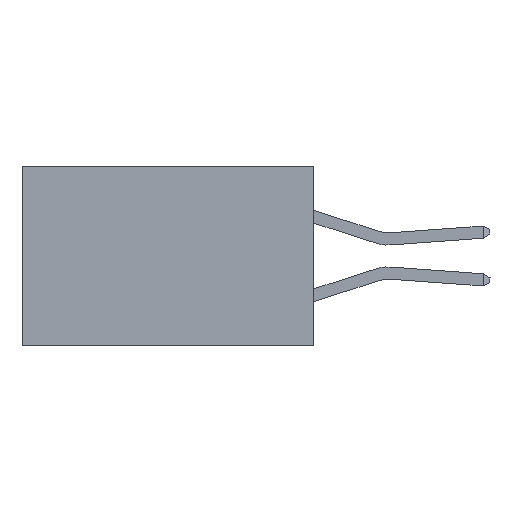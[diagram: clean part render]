
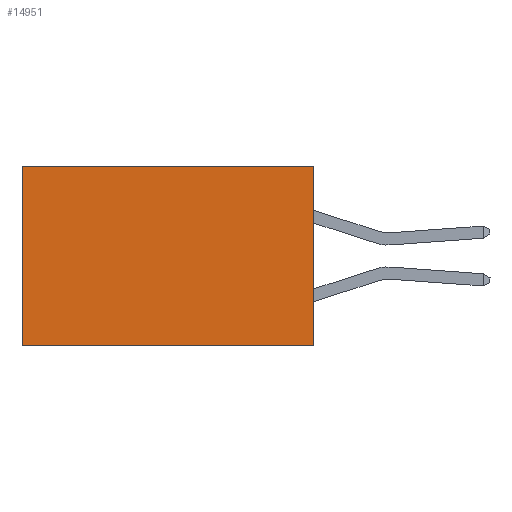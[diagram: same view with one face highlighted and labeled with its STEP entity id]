
A CAD part, left-side view. The second image highlights one B-rep face of the part: STEP entity #14951.
In plain terms, the highlighted planar face has unit normal (-1, 0, 0).
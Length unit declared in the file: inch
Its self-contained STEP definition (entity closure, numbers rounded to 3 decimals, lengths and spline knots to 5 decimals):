
#868 = FACE_OUTER_BOUND ( 'NONE', #6961, .T. ) ;
#1826 = PLANE ( 'NONE',  #11063 ) ;
#2265 = LINE ( 'NONE', #15560, #13310 ) ;
#2710 = ORIENTED_EDGE ( 'NONE', *, *, #5922, .T. ) ;
#3323 = VECTOR ( 'NONE', #17040, 39.37008 ) ;
#3349 = CARTESIAN_POINT ( 'NONE',  ( 0.2875, 0., 0. ) ) ;
#3392 = VERTEX_POINT ( 'NONE', #16728 ) ;
#4278 = VERTEX_POINT ( 'NONE', #12067 ) ;
#4485 = CARTESIAN_POINT ( 'NONE',  ( 0.2875, 0.6, 0. ) ) ;
#5289 = VECTOR ( 'NONE', #5847, 39.37008 ) ;
#5847 = DIRECTION ( 'NONE',  ( 0., 0., -1. ) ) ;
#5922 = EDGE_CURVE ( 'NONE', #6844, #16565, #13421, .T. ) ;
#6163 = DIRECTION ( 'NONE',  ( 1., 0., 0. ) ) ;
#6703 = VECTOR ( 'NONE', #11893, 39.37008 ) ;
#6844 = VERTEX_POINT ( 'NONE', #12405 ) ;
#6961 = EDGE_LOOP ( 'NONE', ( #2710, #13557, #9890, #16768 ) ) ;
#9796 = EDGE_CURVE ( 'NONE', #4278, #3392, #2265, .T. ) ;
#9890 = ORIENTED_EDGE ( 'NONE', *, *, #9796, .F. ) ;
#11063 = AXIS2_PLACEMENT_3D ( 'NONE', #3349, #6163, #16149 ) ;
#11360 = EDGE_CURVE ( 'NONE', #4278, #6844, #17961, .T. ) ;
#11893 = DIRECTION ( 'NONE',  ( 0., 1., 0. ) ) ;
#12067 = CARTESIAN_POINT ( 'NONE',  ( 0.2875, 0., 0. ) ) ;
#12405 = CARTESIAN_POINT ( 'NONE',  ( 0.2875, 0.6, 0. ) ) ;
#12951 = CARTESIAN_POINT ( 'NONE',  ( 0.2875, 0.6, -0.37 ) ) ;
#13151 = EDGE_CURVE ( 'NONE', #3392, #16565, #15154, .T. ) ;
#13291 = CARTESIAN_POINT ( 'NONE',  ( 0.2875, 0., 0. ) ) ;
#13310 = VECTOR ( 'NONE', #16926, 39.37008 ) ;
#13421 = LINE ( 'NONE', #4485, #5289 ) ;
#13557 = ORIENTED_EDGE ( 'NONE', *, *, #13151, .F. ) ;
#14951 = ADVANCED_FACE ( 'NONE', ( #868 ), #1826, .F. ) ;
#15154 = LINE ( 'NONE', #15729, #3323 ) ;
#15560 = CARTESIAN_POINT ( 'NONE',  ( 0.2875, 0., 0. ) ) ;
#15729 = CARTESIAN_POINT ( 'NONE',  ( 0.2875, 0., -0.37 ) ) ;
#16149 = DIRECTION ( 'NONE',  ( 0., 0., -1. ) ) ;
#16565 = VERTEX_POINT ( 'NONE', #12951 ) ;
#16728 = CARTESIAN_POINT ( 'NONE',  ( 0.2875, 0., -0.37 ) ) ;
#16768 = ORIENTED_EDGE ( 'NONE', *, *, #11360, .T. ) ;
#16926 = DIRECTION ( 'NONE',  ( 0., 0., -1. ) ) ;
#17040 = DIRECTION ( 'NONE',  ( 0., 1., 0. ) ) ;
#17961 = LINE ( 'NONE', #13291, #6703 ) ;
